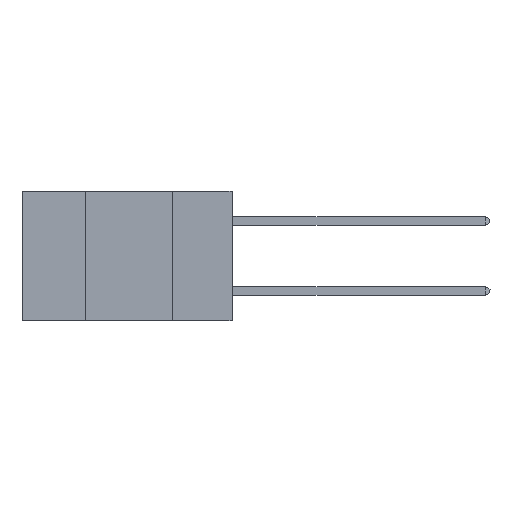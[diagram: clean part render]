
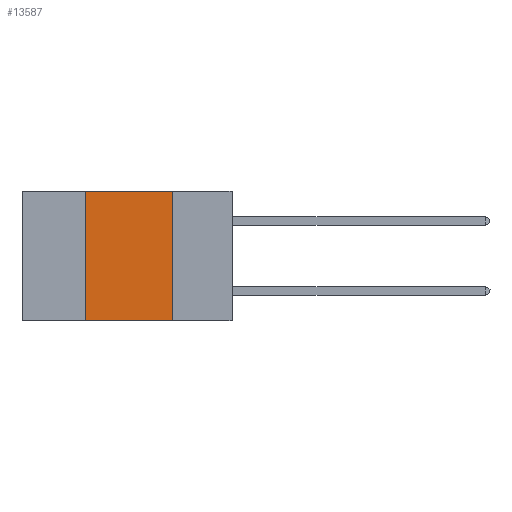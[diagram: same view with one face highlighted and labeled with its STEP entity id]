
A CAD part, left-side view. The second image highlights one B-rep face of the part: STEP entity #13587.
In plain terms, the highlighted planar face has unit normal (-1, 0, 0).
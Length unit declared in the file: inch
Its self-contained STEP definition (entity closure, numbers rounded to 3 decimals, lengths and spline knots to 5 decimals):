
#299 = CARTESIAN_POINT ( 'NONE',  ( 0., 0.6, -0.37 ) ) ;
#442 = EDGE_CURVE ( 'NONE', #7963, #4087, #11141, .T. ) ;
#1004 = ORIENTED_EDGE ( 'NONE', *, *, #9454, .F. ) ;
#1223 = CARTESIAN_POINT ( 'NONE',  ( 0., 0.17, 0. ) ) ;
#1254 = DIRECTION ( 'NONE',  ( 0., 0., -1. ) ) ;
#1811 = VERTEX_POINT ( 'NONE', #7962 ) ;
#1822 = CARTESIAN_POINT ( 'NONE',  ( 0., 0.42, 0. ) ) ;
#1851 = LINE ( 'NONE', #299, #14711 ) ;
#2932 = FACE_OUTER_BOUND ( 'NONE', #5045, .T. ) ;
#2985 = LINE ( 'NONE', #1822, #4737 ) ;
#3595 = EDGE_CURVE ( 'NONE', #1811, #5615, #2985, .T. ) ;
#3966 = CARTESIAN_POINT ( 'NONE',  ( 0., 0.17, 0. ) ) ;
#4087 = VERTEX_POINT ( 'NONE', #13161 ) ;
#4730 = ORIENTED_EDGE ( 'NONE', *, *, #10434, .T. ) ;
#4737 = VECTOR ( 'NONE', #8034, 39.37008 ) ;
#5045 = EDGE_LOOP ( 'NONE', ( #8678, #1004, #7785, #4730 ) ) ;
#5154 = CARTESIAN_POINT ( 'NONE',  ( 0., 0.6, 0. ) ) ;
#5427 = CARTESIAN_POINT ( 'NONE',  ( 0., 0.6, 0. ) ) ;
#5615 = VERTEX_POINT ( 'NONE', #14918 ) ;
#6960 = DIRECTION ( 'NONE',  ( 0., -1., 0. ) ) ;
#7460 = PLANE ( 'NONE',  #9476 ) ;
#7741 = VECTOR ( 'NONE', #6960, 39.37008 ) ;
#7785 = ORIENTED_EDGE ( 'NONE', *, *, #3595, .F. ) ;
#7962 = CARTESIAN_POINT ( 'NONE',  ( 0., 0.42, -0.37 ) ) ;
#7963 = VERTEX_POINT ( 'NONE', #1223 ) ;
#8034 = DIRECTION ( 'NONE',  ( 0., 0., 1. ) ) ;
#8678 = ORIENTED_EDGE ( 'NONE', *, *, #442, .F. ) ;
#8697 = DIRECTION ( 'NONE',  ( 1., 0., 0. ) ) ;
#9197 = DIRECTION ( 'NONE',  ( 0., -1., 0. ) ) ;
#9454 = EDGE_CURVE ( 'NONE', #5615, #7963, #11041, .T. ) ;
#9476 = AXIS2_PLACEMENT_3D ( 'NONE', #5154, #8697, #1254 ) ;
#10378 = VECTOR ( 'NONE', #12703, 39.37008 ) ;
#10434 = EDGE_CURVE ( 'NONE', #1811, #4087, #1851, .T. ) ;
#11041 = LINE ( 'NONE', #5427, #7741 ) ;
#11141 = LINE ( 'NONE', #3966, #10378 ) ;
#12703 = DIRECTION ( 'NONE',  ( 0., 0., -1. ) ) ;
#13161 = CARTESIAN_POINT ( 'NONE',  ( 0., 0.17, -0.37 ) ) ;
#13587 = ADVANCED_FACE ( 'NONE', ( #2932 ), #7460, .F. ) ;
#14711 = VECTOR ( 'NONE', #9197, 39.37008 ) ;
#14918 = CARTESIAN_POINT ( 'NONE',  ( 0., 0.42, 0. ) ) ;
